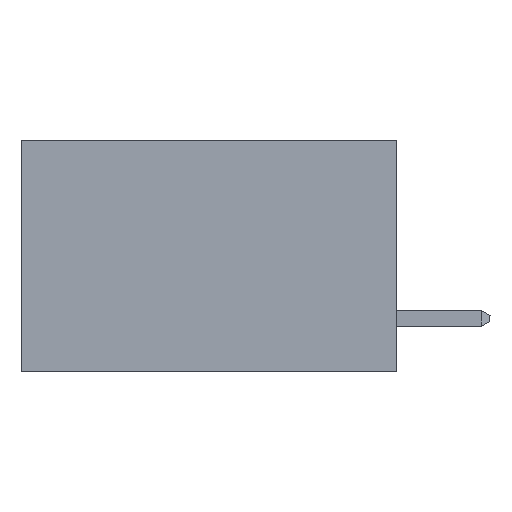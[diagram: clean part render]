
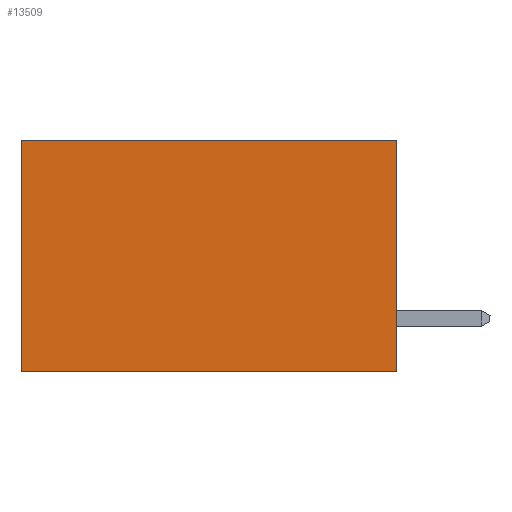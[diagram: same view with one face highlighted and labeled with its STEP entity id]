
A CAD part, left-side view. The second image highlights one B-rep face of the part: STEP entity #13509.
In plain terms, the highlighted planar face has unit normal (-1, 0, 0).
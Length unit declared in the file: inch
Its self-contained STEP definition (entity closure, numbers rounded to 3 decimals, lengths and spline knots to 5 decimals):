
#32 = VERTEX_POINT ( 'NONE', #10074 ) ;
#321 = LINE ( 'NONE', #4473, #19109 ) ;
#464 = DIRECTION ( 'NONE',  ( 0., 0., -1. ) ) ;
#865 = EDGE_CURVE ( 'NONE', #32, #20697, #321, .T. ) ;
#1377 = VECTOR ( 'NONE', #2071, 39.37008 ) ;
#1948 = LINE ( 'NONE', #23286, #1377 ) ;
#2071 = DIRECTION ( 'NONE',  ( 0., 1., 0. ) ) ;
#3157 = CARTESIAN_POINT ( 'NONE',  ( 0.298, 0., -0.37 ) ) ;
#4157 = PLANE ( 'NONE',  #17382 ) ;
#4473 = CARTESIAN_POINT ( 'NONE',  ( 0.298, 0., 0. ) ) ;
#4476 = ORIENTED_EDGE ( 'NONE', *, *, #865, .F. ) ;
#5685 = CARTESIAN_POINT ( 'NONE',  ( 0.298, 0.6, 0. ) ) ;
#6289 = VECTOR ( 'NONE', #21396, 39.37008 ) ;
#6951 = ORIENTED_EDGE ( 'NONE', *, *, #7107, .T. ) ;
#7107 = EDGE_CURVE ( 'NONE', #32, #17678, #1948, .T. ) ;
#8210 = CARTESIAN_POINT ( 'NONE',  ( 0.298, 0., -0.37 ) ) ;
#9525 = CARTESIAN_POINT ( 'NONE',  ( 0.298, 0., 0. ) ) ;
#9961 = LINE ( 'NONE', #12507, #6289 ) ;
#10074 = CARTESIAN_POINT ( 'NONE',  ( 0.298, 0., 0. ) ) ;
#11726 = DIRECTION ( 'NONE',  ( 0., 0., -1. ) ) ;
#12507 = CARTESIAN_POINT ( 'NONE',  ( 0.298, 0.6, 0. ) ) ;
#13005 = DIRECTION ( 'NONE',  ( 1., 0., 0. ) ) ;
#13509 = ADVANCED_FACE ( 'NONE', ( #22321 ), #4157, .F. ) ;
#14425 = LINE ( 'NONE', #3157, #17552 ) ;
#14822 = VERTEX_POINT ( 'NONE', #20423 ) ;
#15255 = EDGE_CURVE ( 'NONE', #17678, #14822, #9961, .T. ) ;
#15574 = ORIENTED_EDGE ( 'NONE', *, *, #16616, .F. ) ;
#16616 = EDGE_CURVE ( 'NONE', #20697, #14822, #14425, .T. ) ;
#17382 = AXIS2_PLACEMENT_3D ( 'NONE', #9525, #13005, #464 ) ;
#17552 = VECTOR ( 'NONE', #19525, 39.37008 ) ;
#17678 = VERTEX_POINT ( 'NONE', #5685 ) ;
#17948 = ORIENTED_EDGE ( 'NONE', *, *, #15255, .T. ) ;
#19109 = VECTOR ( 'NONE', #11726, 39.37008 ) ;
#19525 = DIRECTION ( 'NONE',  ( 0., 1., 0. ) ) ;
#19612 = EDGE_LOOP ( 'NONE', ( #17948, #15574, #4476, #6951 ) ) ;
#20423 = CARTESIAN_POINT ( 'NONE',  ( 0.298, 0.6, -0.37 ) ) ;
#20697 = VERTEX_POINT ( 'NONE', #8210 ) ;
#21396 = DIRECTION ( 'NONE',  ( 0., 0., -1. ) ) ;
#22321 = FACE_OUTER_BOUND ( 'NONE', #19612, .T. ) ;
#23286 = CARTESIAN_POINT ( 'NONE',  ( 0.298, 0., 0. ) ) ;
